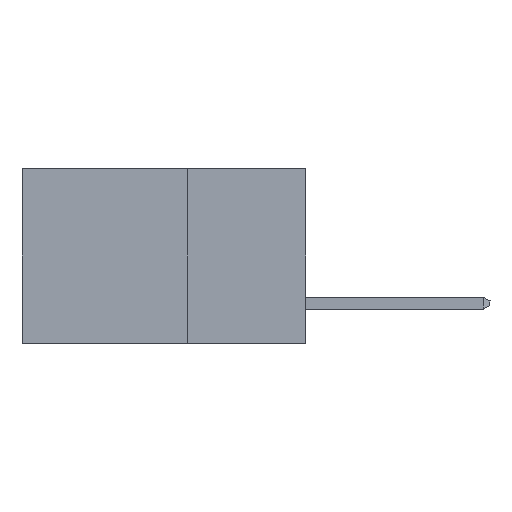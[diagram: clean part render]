
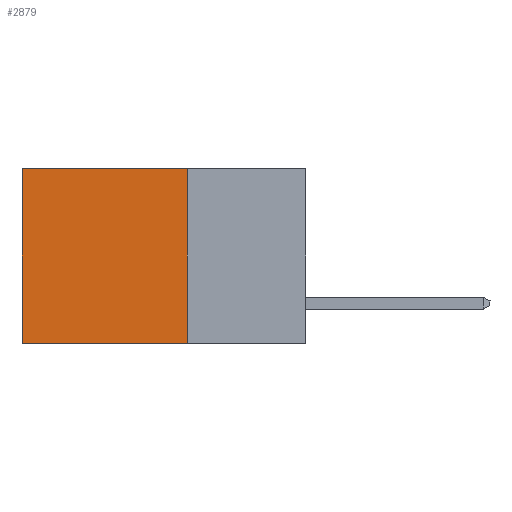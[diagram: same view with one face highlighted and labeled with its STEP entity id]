
A CAD part, left-side view. The second image highlights one B-rep face of the part: STEP entity #2879.
In plain terms, the highlighted planar face has unit normal (-1, 0, 0).
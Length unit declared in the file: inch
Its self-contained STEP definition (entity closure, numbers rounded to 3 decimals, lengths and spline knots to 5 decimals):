
#9 = FACE_OUTER_BOUND ( 'NONE', #746, .T. ) ;
#47 = LINE ( 'NONE', #11370, #11838 ) ;
#279 = ORIENTED_EDGE ( 'NONE', *, *, #3468, .F. ) ;
#381 = CARTESIAN_POINT ( 'NONE',  ( 0.298, 0.25, 0. ) ) ;
#585 = ORIENTED_EDGE ( 'NONE', *, *, #5668, .F. ) ;
#645 = VERTEX_POINT ( 'NONE', #9227 ) ;
#746 = EDGE_LOOP ( 'NONE', ( #2488, #279, #585, #3463 ) ) ;
#1836 = AXIS2_PLACEMENT_3D ( 'NONE', #8121, #7012, #6012 ) ;
#2488 = ORIENTED_EDGE ( 'NONE', *, *, #9725, .T. ) ;
#2879 = ADVANCED_FACE ( 'NONE', ( #9 ), #9090, .F. ) ;
#2965 = LINE ( 'NONE', #12791, #5597 ) ;
#3463 = ORIENTED_EDGE ( 'NONE', *, *, #10131, .T. ) ;
#3468 = EDGE_CURVE ( 'NONE', #12427, #645, #2965, .T. ) ;
#4911 = CARTESIAN_POINT ( 'NONE',  ( 0.298, 0.25, -0.37 ) ) ;
#5597 = VECTOR ( 'NONE', #11011, 39.37008 ) ;
#5618 = LINE ( 'NONE', #381, #7179 ) ;
#5668 = EDGE_CURVE ( 'NONE', #7741, #12427, #12405, .T. ) ;
#6012 = DIRECTION ( 'NONE',  ( 0., 0., -1. ) ) ;
#6243 = DIRECTION ( 'NONE',  ( 0., 1., 0. ) ) ;
#6470 = DIRECTION ( 'NONE',  ( 0., 0., -1. ) ) ;
#7012 = DIRECTION ( 'NONE',  ( 1., 0., 0. ) ) ;
#7179 = VECTOR ( 'NONE', #6243, 39.37008 ) ;
#7741 = VERTEX_POINT ( 'NONE', #9407 ) ;
#8121 = CARTESIAN_POINT ( 'NONE',  ( 0.298, 0.25, 0. ) ) ;
#9011 = DIRECTION ( 'NONE',  ( 0., 0., -1. ) ) ;
#9090 = PLANE ( 'NONE',  #1836 ) ;
#9227 = CARTESIAN_POINT ( 'NONE',  ( 0.298, 0.6, -0.37 ) ) ;
#9407 = CARTESIAN_POINT ( 'NONE',  ( 0.298, 0.25, 0. ) ) ;
#9725 = EDGE_CURVE ( 'NONE', #12645, #645, #47, .T. ) ;
#10049 = CARTESIAN_POINT ( 'NONE',  ( 0.298, 0.25, 0. ) ) ;
#10131 = EDGE_CURVE ( 'NONE', #7741, #12645, #5618, .T. ) ;
#11011 = DIRECTION ( 'NONE',  ( 0., 1., 0. ) ) ;
#11370 = CARTESIAN_POINT ( 'NONE',  ( 0.298, 0.6, 0. ) ) ;
#11838 = VECTOR ( 'NONE', #6470, 39.37008 ) ;
#12087 = VECTOR ( 'NONE', #9011, 39.37008 ) ;
#12182 = CARTESIAN_POINT ( 'NONE',  ( 0.298, 0.6, 0. ) ) ;
#12405 = LINE ( 'NONE', #10049, #12087 ) ;
#12427 = VERTEX_POINT ( 'NONE', #4911 ) ;
#12645 = VERTEX_POINT ( 'NONE', #12182 ) ;
#12791 = CARTESIAN_POINT ( 'NONE',  ( 0.298, 0.25, -0.37 ) ) ;
